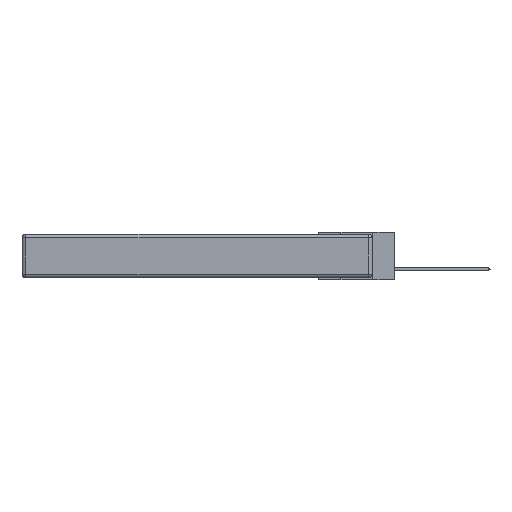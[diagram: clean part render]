
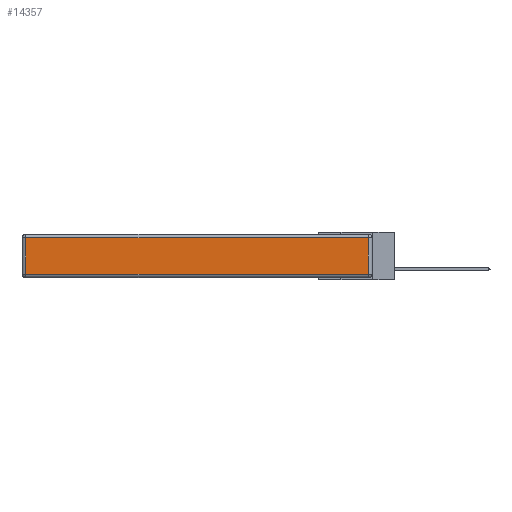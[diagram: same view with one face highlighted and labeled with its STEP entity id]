
A CAD part, left-side view. The second image highlights one B-rep face of the part: STEP entity #14357.
In plain terms, the highlighted planar face has unit normal (-1, 0, 0).
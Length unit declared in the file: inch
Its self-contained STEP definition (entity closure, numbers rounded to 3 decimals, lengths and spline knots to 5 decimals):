
#126 = LINE ( 'NONE', #13700, #16625 ) ;
#464 = EDGE_CURVE ( 'NONE', #2513, #16722, #3804, .T. ) ;
#529 = FACE_OUTER_BOUND ( 'NONE', #5914, .T. ) ;
#604 = ORIENTED_EDGE ( 'NONE', *, *, #464, .T. ) ;
#2513 = VERTEX_POINT ( 'NONE', #6308 ) ;
#2611 = CARTESIAN_POINT ( 'NONE',  ( 0., 0., -0.343 ) ) ;
#3804 = LINE ( 'NONE', #4285, #10973 ) ;
#3958 = LINE ( 'NONE', #7922, #13295 ) ;
#4199 = AXIS2_PLACEMENT_3D ( 'NONE', #2611, #6590, #9534 ) ;
#4285 = CARTESIAN_POINT ( 'NONE',  ( 0., 2.72, -0.343 ) ) ;
#4330 = ORIENTED_EDGE ( 'NONE', *, *, #8122, .T. ) ;
#5914 = EDGE_LOOP ( 'NONE', ( #13774, #13352, #4330, #604 ) ) ;
#6159 = CARTESIAN_POINT ( 'NONE',  ( 0., 0.03, -0.03 ) ) ;
#6308 = CARTESIAN_POINT ( 'NONE',  ( 0., 2.72, -0.03 ) ) ;
#6590 = DIRECTION ( 'NONE',  ( -1., 0., 0. ) ) ;
#6996 = VERTEX_POINT ( 'NONE', #11919 ) ;
#7922 = CARTESIAN_POINT ( 'NONE',  ( 0., 0.03, -0.343 ) ) ;
#8122 = EDGE_CURVE ( 'NONE', #15768, #2513, #126, .T. ) ;
#8828 = VECTOR ( 'NONE', #10695, 39.37008 ) ;
#9534 = DIRECTION ( 'NONE',  ( 0., 0., 1. ) ) ;
#10371 = EDGE_CURVE ( 'NONE', #16722, #6996, #15153, .T. ) ;
#10695 = DIRECTION ( 'NONE',  ( 0., -1., 0. ) ) ;
#10973 = VECTOR ( 'NONE', #16720, 39.37008 ) ;
#10982 = DIRECTION ( 'NONE',  ( 0., 1., 0. ) ) ;
#11919 = CARTESIAN_POINT ( 'NONE',  ( 0., 0.03, -0.313 ) ) ;
#12229 = DIRECTION ( 'NONE',  ( 0., 0., 1. ) ) ;
#13295 = VECTOR ( 'NONE', #12229, 39.37008 ) ;
#13352 = ORIENTED_EDGE ( 'NONE', *, *, #16567, .T. ) ;
#13700 = CARTESIAN_POINT ( 'NONE',  ( 0., 2.75, -0.03 ) ) ;
#13774 = ORIENTED_EDGE ( 'NONE', *, *, #10371, .T. ) ;
#14357 = ADVANCED_FACE ( 'NONE', ( #529 ), #16349, .T. ) ;
#15153 = LINE ( 'NONE', #17741, #8828 ) ;
#15254 = CARTESIAN_POINT ( 'NONE',  ( 0., 2.72, -0.313 ) ) ;
#15768 = VERTEX_POINT ( 'NONE', #6159 ) ;
#16349 = PLANE ( 'NONE',  #4199 ) ;
#16567 = EDGE_CURVE ( 'NONE', #6996, #15768, #3958, .T. ) ;
#16625 = VECTOR ( 'NONE', #10982, 39.37008 ) ;
#16720 = DIRECTION ( 'NONE',  ( 0., 0., -1. ) ) ;
#16722 = VERTEX_POINT ( 'NONE', #15254 ) ;
#17741 = CARTESIAN_POINT ( 'NONE',  ( 0., 0., -0.313 ) ) ;
